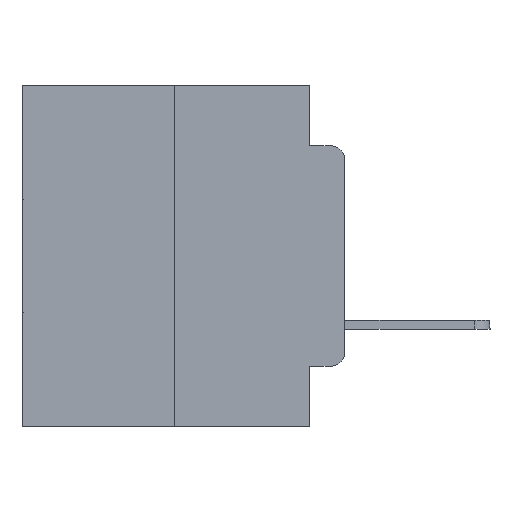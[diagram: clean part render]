
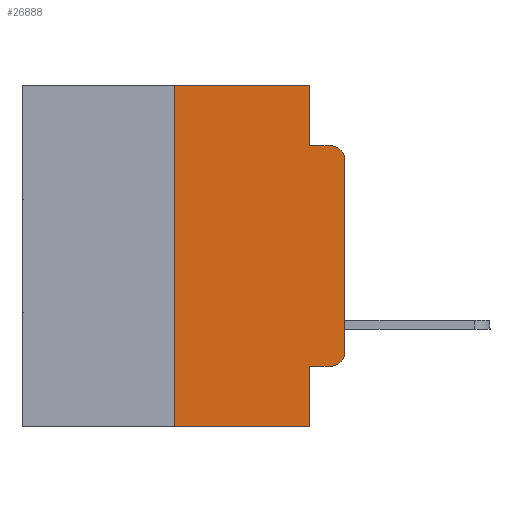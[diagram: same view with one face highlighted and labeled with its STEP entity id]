
A CAD part, left-side view. The second image highlights one B-rep face of the part: STEP entity #26888.
In plain terms, the highlighted planar face has unit normal (-1, 0, 0).
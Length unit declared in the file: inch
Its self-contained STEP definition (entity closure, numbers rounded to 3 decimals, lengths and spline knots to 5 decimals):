
#43 = ORIENTED_EDGE ( 'NONE', *, *, #10159, .T. ) ;
#206 = DIRECTION ( 'NONE',  ( 0., 0., -1. ) ) ;
#1811 = CARTESIAN_POINT ( 'NONE',  ( 0., 0.25, 0. ) ) ;
#2355 = CARTESIAN_POINT ( 'NONE',  ( 0., 0.02, -0.1085 ) ) ;
#2478 = ORIENTED_EDGE ( 'NONE', *, *, #4399, .T. ) ;
#3006 = ORIENTED_EDGE ( 'NONE', *, *, #5338, .T. ) ;
#3864 = CIRCLE ( 'NONE', #11201, 0.02 ) ;
#4068 = VECTOR ( 'NONE', #4724, 39.37008 ) ;
#4358 = VECTOR ( 'NONE', #8864, 39.37008 ) ;
#4399 = EDGE_CURVE ( 'NONE', #7399, #15674, #12062, .T. ) ;
#4724 = DIRECTION ( 'NONE',  ( 0., -1., 0. ) ) ;
#5266 = DIRECTION ( 'NONE',  ( 0., 0., -1. ) ) ;
#5338 = EDGE_CURVE ( 'NONE', #15674, #9302, #15058, .T. ) ;
#5748 = VERTEX_POINT ( 'NONE', #7066 ) ;
#5817 = VERTEX_POINT ( 'NONE', #13259 ) ;
#6046 = VECTOR ( 'NONE', #6921, 39.37008 ) ;
#6921 = DIRECTION ( 'NONE',  ( 0., 0., -1. ) ) ;
#7066 = CARTESIAN_POINT ( 'NONE',  ( 0., 0.25, -0.5 ) ) ;
#7399 = VERTEX_POINT ( 'NONE', #25114 ) ;
#8437 = AXIS2_PLACEMENT_3D ( 'NONE', #27528, #27666, #5266 ) ;
#8536 = CARTESIAN_POINT ( 'NONE',  ( 0., 0.473, 0. ) ) ;
#8864 = DIRECTION ( 'NONE',  ( 0., 0., 1. ) ) ;
#9229 = CARTESIAN_POINT ( 'NONE',  ( 0., 0.02, -0.3915 ) ) ;
#9302 = VERTEX_POINT ( 'NONE', #14741 ) ;
#9894 = CARTESIAN_POINT ( 'NONE',  ( 0., 0.051, -0.0885 ) ) ;
#10159 = EDGE_CURVE ( 'NONE', #5748, #5817, #11336, .T. ) ;
#10233 = AXIS2_PLACEMENT_3D ( 'NONE', #9229, #13541, #24442 ) ;
#11012 = EDGE_LOOP ( 'NONE', ( #3006, #19416, #18821, #23500, #24014, #23160, #43, #24851, #16069, #2478 ) ) ;
#11118 = DIRECTION ( 'NONE',  ( -1., 0., 0. ) ) ;
#11201 = AXIS2_PLACEMENT_3D ( 'NONE', #2355, #11118, #206 ) ;
#11235 = CARTESIAN_POINT ( 'NONE',  ( 0., 0.02, -0.0885 ) ) ;
#11289 = EDGE_CURVE ( 'NONE', #21197, #26449, #28214, .T. ) ;
#11336 = LINE ( 'NONE', #15215, #4068 ) ;
#12060 = LINE ( 'NONE', #14648, #20805 ) ;
#12062 = CIRCLE ( 'NONE', #10233, 0.02 ) ;
#13137 = DIRECTION ( 'NONE',  ( 0., -1., 0. ) ) ;
#13259 = CARTESIAN_POINT ( 'NONE',  ( 0., 0.051, -0.5 ) ) ;
#13541 = DIRECTION ( 'NONE',  ( -1., 0., 0. ) ) ;
#13659 = CARTESIAN_POINT ( 'NONE',  ( 0., 0., 0. ) ) ;
#13956 = CARTESIAN_POINT ( 'NONE',  ( 0., 0.051, 0. ) ) ;
#14429 = EDGE_CURVE ( 'NONE', #9302, #19626, #3864, .T. ) ;
#14648 = CARTESIAN_POINT ( 'NONE',  ( 0., 0.051, -0.0885 ) ) ;
#14741 = CARTESIAN_POINT ( 'NONE',  ( 0., 0., -0.1085 ) ) ;
#15058 = LINE ( 'NONE', #13659, #4358 ) ;
#15206 = VECTOR ( 'NONE', #26193, 39.37008 ) ;
#15215 = CARTESIAN_POINT ( 'NONE',  ( 0., 0.473, -0.5 ) ) ;
#15674 = VERTEX_POINT ( 'NONE', #26374 ) ;
#16019 = VECTOR ( 'NONE', #27142, 39.37008 ) ;
#16069 = ORIENTED_EDGE ( 'NONE', *, *, #26402, .T. ) ;
#16599 = CARTESIAN_POINT ( 'NONE',  ( 0., 0.051, -0.4115 ) ) ;
#16795 = LINE ( 'NONE', #18808, #24914 ) ;
#17982 = LINE ( 'NONE', #13956, #6046 ) ;
#18381 = CARTESIAN_POINT ( 'NONE',  ( 0., 0.051, 0. ) ) ;
#18522 = CARTESIAN_POINT ( 'NONE',  ( 0., 0.25, 0. ) ) ;
#18773 = FACE_OUTER_BOUND ( 'NONE', #11012, .T. ) ;
#18808 = CARTESIAN_POINT ( 'NONE',  ( 0., 0.051, -0.4115 ) ) ;
#18821 = ORIENTED_EDGE ( 'NONE', *, *, #26469, .F. ) ;
#19416 = ORIENTED_EDGE ( 'NONE', *, *, #14429, .T. ) ;
#19626 = VERTEX_POINT ( 'NONE', #11235 ) ;
#20523 = LINE ( 'NONE', #18381, #16019 ) ;
#20805 = VECTOR ( 'NONE', #20819, 39.37008 ) ;
#20819 = DIRECTION ( 'NONE',  ( 0., -1., 0. ) ) ;
#21197 = VERTEX_POINT ( 'NONE', #18522 ) ;
#21280 = EDGE_CURVE ( 'NONE', #25921, #5817, #20523, .T. ) ;
#22079 = VECTOR ( 'NONE', #13137, 39.37008 ) ;
#23160 = ORIENTED_EDGE ( 'NONE', *, *, #24774, .F. ) ;
#23500 = ORIENTED_EDGE ( 'NONE', *, *, #25267, .F. ) ;
#24014 = ORIENTED_EDGE ( 'NONE', *, *, #11289, .F. ) ;
#24027 = VERTEX_POINT ( 'NONE', #9894 ) ;
#24442 = DIRECTION ( 'NONE',  ( 0., 0., -1. ) ) ;
#24774 = EDGE_CURVE ( 'NONE', #5748, #21197, #28206, .T. ) ;
#24851 = ORIENTED_EDGE ( 'NONE', *, *, #21280, .F. ) ;
#24914 = VECTOR ( 'NONE', #25122, 39.37008 ) ;
#24942 = PLANE ( 'NONE',  #8437 ) ;
#25114 = CARTESIAN_POINT ( 'NONE',  ( 0., 0.02, -0.4115 ) ) ;
#25122 = DIRECTION ( 'NONE',  ( 0., -1., 0. ) ) ;
#25267 = EDGE_CURVE ( 'NONE', #26449, #24027, #17982, .T. ) ;
#25921 = VERTEX_POINT ( 'NONE', #16599 ) ;
#26193 = DIRECTION ( 'NONE',  ( 0., 0., 1. ) ) ;
#26374 = CARTESIAN_POINT ( 'NONE',  ( 0., 0., -0.3915 ) ) ;
#26402 = EDGE_CURVE ( 'NONE', #25921, #7399, #16795, .T. ) ;
#26449 = VERTEX_POINT ( 'NONE', #27418 ) ;
#26469 = EDGE_CURVE ( 'NONE', #24027, #19626, #12060, .T. ) ;
#26888 = ADVANCED_FACE ( 'NONE', ( #18773 ), #24942, .F. ) ;
#27142 = DIRECTION ( 'NONE',  ( 0., 0., -1. ) ) ;
#27418 = CARTESIAN_POINT ( 'NONE',  ( 0., 0.051, 0. ) ) ;
#27528 = CARTESIAN_POINT ( 'NONE',  ( 0., 0.473, 0. ) ) ;
#27666 = DIRECTION ( 'NONE',  ( 1., 0., 0. ) ) ;
#28206 = LINE ( 'NONE', #1811, #15206 ) ;
#28214 = LINE ( 'NONE', #8536, #22079 ) ;
